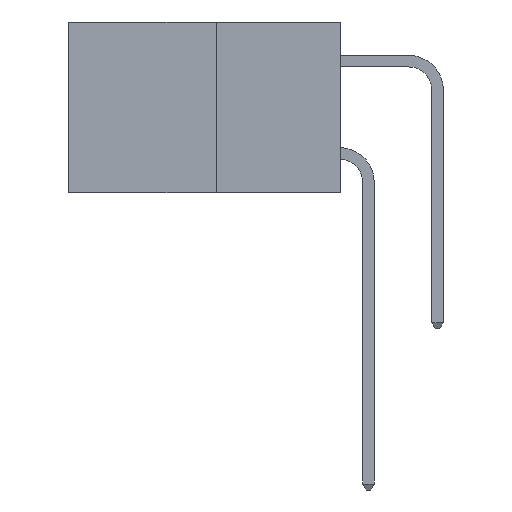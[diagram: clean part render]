
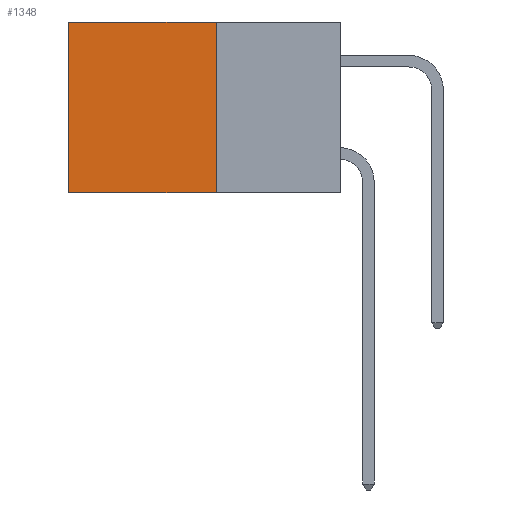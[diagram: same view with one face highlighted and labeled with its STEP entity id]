
A CAD part, left-side view. The second image highlights one B-rep face of the part: STEP entity #1348.
In plain terms, the highlighted planar face has unit normal (-1, 0, 0).
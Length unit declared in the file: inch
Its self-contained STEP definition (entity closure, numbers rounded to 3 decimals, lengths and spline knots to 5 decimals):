
#26 = VECTOR ( 'NONE', #633, 39.37008 ) ;
#291 = CARTESIAN_POINT ( 'NONE',  ( 0.277, 0.59, 0. ) ) ;
#487 = ORIENTED_EDGE ( 'NONE', *, *, #27898, .F. ) ;
#633 = DIRECTION ( 'NONE',  ( 0., 0., -1. ) ) ;
#1059 = DIRECTION ( 'NONE',  ( 0., 0., -1. ) ) ;
#1348 = ADVANCED_FACE ( 'NONE', ( #22430 ), #5573, .F. ) ;
#1605 = LINE ( 'NONE', #6473, #20468 ) ;
#2391 = CARTESIAN_POINT ( 'NONE',  ( 0.277, 0.27, 0. ) ) ;
#3360 = DIRECTION ( 'NONE',  ( 0., 0., -1. ) ) ;
#3519 = DIRECTION ( 'NONE',  ( 1., 0., 0. ) ) ;
#5365 = CARTESIAN_POINT ( 'NONE',  ( 0.277, 0.27, -0.37 ) ) ;
#5573 = PLANE ( 'NONE',  #16640 ) ;
#6473 = CARTESIAN_POINT ( 'NONE',  ( 0.277, 0.27, 0. ) ) ;
#8721 = CARTESIAN_POINT ( 'NONE',  ( 0.277, 0.27, -0.37 ) ) ;
#9798 = VERTEX_POINT ( 'NONE', #2391 ) ;
#10296 = ORIENTED_EDGE ( 'NONE', *, *, #16598, .T. ) ;
#10965 = CARTESIAN_POINT ( 'NONE',  ( 0.277, 0.59, -0.37 ) ) ;
#11485 = VECTOR ( 'NONE', #1059, 39.37008 ) ;
#12497 = CARTESIAN_POINT ( 'NONE',  ( 0.277, 0.27, -0.37 ) ) ;
#16598 = EDGE_CURVE ( 'NONE', #9798, #29724, #1605, .T. ) ;
#16640 = AXIS2_PLACEMENT_3D ( 'NONE', #5365, #3519, #3360 ) ;
#20468 = VECTOR ( 'NONE', #31726, 39.37008 ) ;
#20478 = ORIENTED_EDGE ( 'NONE', *, *, #22077, .T. ) ;
#20570 = LINE ( 'NONE', #10965, #26 ) ;
#21629 = LINE ( 'NONE', #8721, #27541 ) ;
#22077 = EDGE_CURVE ( 'NONE', #29724, #22863, #20570, .T. ) ;
#22430 = FACE_OUTER_BOUND ( 'NONE', #31164, .T. ) ;
#22863 = VERTEX_POINT ( 'NONE', #23921 ) ;
#23921 = CARTESIAN_POINT ( 'NONE',  ( 0.277, 0.59, -0.37 ) ) ;
#24439 = EDGE_CURVE ( 'NONE', #9798, #30924, #24986, .T. ) ;
#24986 = LINE ( 'NONE', #31566, #11485 ) ;
#25392 = ORIENTED_EDGE ( 'NONE', *, *, #24439, .F. ) ;
#26611 = DIRECTION ( 'NONE',  ( 0., 1., 0. ) ) ;
#27541 = VECTOR ( 'NONE', #26611, 39.37008 ) ;
#27898 = EDGE_CURVE ( 'NONE', #30924, #22863, #21629, .T. ) ;
#29724 = VERTEX_POINT ( 'NONE', #291 ) ;
#30924 = VERTEX_POINT ( 'NONE', #12497 ) ;
#31164 = EDGE_LOOP ( 'NONE', ( #20478, #487, #25392, #10296 ) ) ;
#31566 = CARTESIAN_POINT ( 'NONE',  ( 0.277, 0.27, -0.37 ) ) ;
#31726 = DIRECTION ( 'NONE',  ( 0., 1., 0. ) ) ;
